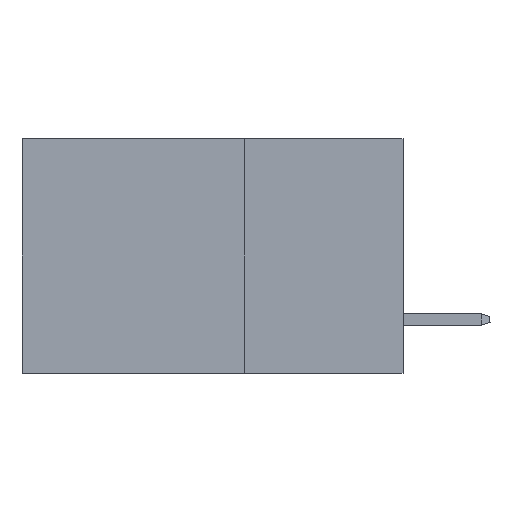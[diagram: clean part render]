
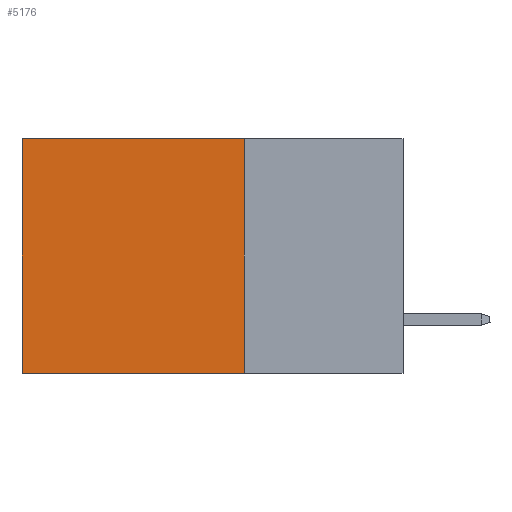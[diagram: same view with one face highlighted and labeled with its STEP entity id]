
A CAD part, left-side view. The second image highlights one B-rep face of the part: STEP entity #5176.
In plain terms, the highlighted planar face has unit normal (-1, 0, 0).
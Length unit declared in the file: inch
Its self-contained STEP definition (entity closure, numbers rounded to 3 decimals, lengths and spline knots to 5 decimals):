
#1045 = EDGE_CURVE ( 'NONE', #19633, #5188, #13549, .T. ) ;
#1736 = CARTESIAN_POINT ( 'NONE',  ( 0.2875, 0.25, 0. ) ) ;
#1971 = EDGE_CURVE ( 'NONE', #17245, #21399, #17462, .T. ) ;
#2099 = DIRECTION ( 'NONE',  ( 0., 0., -1. ) ) ;
#2530 = DIRECTION ( 'NONE',  ( 0., 1., 0. ) ) ;
#3261 = CARTESIAN_POINT ( 'NONE',  ( 0.2875, 0.6, -0.37 ) ) ;
#4016 = CARTESIAN_POINT ( 'NONE',  ( 0.2875, 0.6, 0. ) ) ;
#4975 = CARTESIAN_POINT ( 'NONE',  ( 0.2875, 0.25, 0. ) ) ;
#5015 = EDGE_CURVE ( 'NONE', #17245, #19633, #12640, .T. ) ;
#5176 = ADVANCED_FACE ( 'NONE', ( #17200 ), #18759, .F. ) ;
#5188 = VERTEX_POINT ( 'NONE', #3261 ) ;
#5721 = ORIENTED_EDGE ( 'NONE', *, *, #1045, .F. ) ;
#6147 = ORIENTED_EDGE ( 'NONE', *, *, #21882, .T. ) ;
#6411 = VECTOR ( 'NONE', #21767, 39.37008 ) ;
#6432 = DIRECTION ( 'NONE',  ( 0., 1., 0. ) ) ;
#8591 = ORIENTED_EDGE ( 'NONE', *, *, #5015, .F. ) ;
#9275 = LINE ( 'NONE', #4016, #18200 ) ;
#11672 = CARTESIAN_POINT ( 'NONE',  ( 0.2875, 0.25, 0. ) ) ;
#12640 = LINE ( 'NONE', #1736, #6411 ) ;
#12936 = CARTESIAN_POINT ( 'NONE',  ( 0.2875, 0.25, -0.37 ) ) ;
#13549 = LINE ( 'NONE', #15135, #19650 ) ;
#13896 = EDGE_LOOP ( 'NONE', ( #6147, #5721, #8591, #20672 ) ) ;
#15135 = CARTESIAN_POINT ( 'NONE',  ( 0.2875, 0.25, -0.37 ) ) ;
#16370 = AXIS2_PLACEMENT_3D ( 'NONE', #11672, #19113, #20547 ) ;
#16760 = CARTESIAN_POINT ( 'NONE',  ( 0.2875, 0.6, 0. ) ) ;
#17200 = FACE_OUTER_BOUND ( 'NONE', #13896, .T. ) ;
#17245 = VERTEX_POINT ( 'NONE', #21154 ) ;
#17462 = LINE ( 'NONE', #4975, #19684 ) ;
#18200 = VECTOR ( 'NONE', #2099, 39.37008 ) ;
#18759 = PLANE ( 'NONE',  #16370 ) ;
#19113 = DIRECTION ( 'NONE',  ( 1., 0., 0. ) ) ;
#19633 = VERTEX_POINT ( 'NONE', #12936 ) ;
#19650 = VECTOR ( 'NONE', #2530, 39.37008 ) ;
#19684 = VECTOR ( 'NONE', #6432, 39.37008 ) ;
#20547 = DIRECTION ( 'NONE',  ( 0., 0., -1. ) ) ;
#20672 = ORIENTED_EDGE ( 'NONE', *, *, #1971, .T. ) ;
#21154 = CARTESIAN_POINT ( 'NONE',  ( 0.2875, 0.25, 0. ) ) ;
#21399 = VERTEX_POINT ( 'NONE', #16760 ) ;
#21767 = DIRECTION ( 'NONE',  ( 0., 0., -1. ) ) ;
#21882 = EDGE_CURVE ( 'NONE', #21399, #5188, #9275, .T. ) ;
